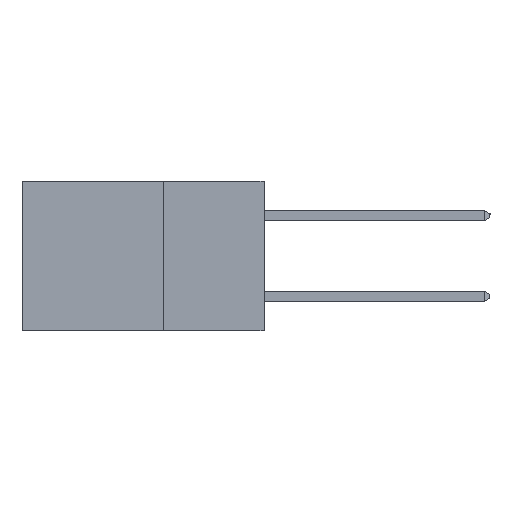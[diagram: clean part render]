
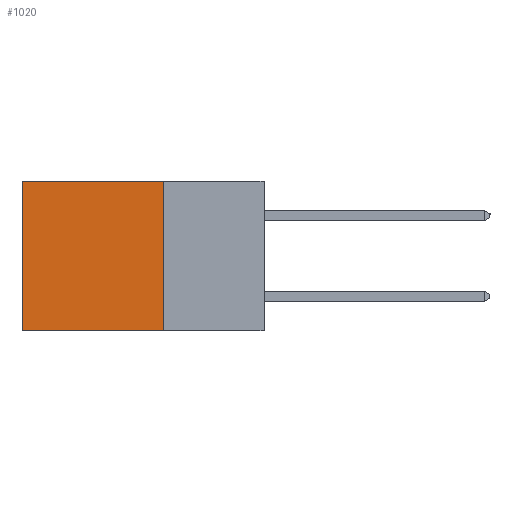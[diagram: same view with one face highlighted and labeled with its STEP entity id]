
A CAD part, left-side view. The second image highlights one B-rep face of the part: STEP entity #1020.
In plain terms, the highlighted planar face has unit normal (-1, 0, 0).
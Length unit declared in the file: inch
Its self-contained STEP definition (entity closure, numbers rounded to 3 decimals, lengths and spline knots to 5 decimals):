
#186 = VERTEX_POINT ( 'NONE', #15133 ) ;
#246 = VERTEX_POINT ( 'NONE', #11423 ) ;
#358 = AXIS2_PLACEMENT_3D ( 'NONE', #12783, #1730, #6645 ) ;
#474 = VECTOR ( 'NONE', #1845, 39.37008 ) ;
#616 = VECTOR ( 'NONE', #12439, 39.37008 ) ;
#1020 = ADVANCED_FACE ( 'NONE', ( #1878 ), #7836, .F. ) ;
#1242 = VECTOR ( 'NONE', #9492, 39.37008 ) ;
#1294 = EDGE_CURVE ( 'NONE', #246, #11935, #6142, .T. ) ;
#1351 = VERTEX_POINT ( 'NONE', #8967 ) ;
#1730 = DIRECTION ( 'NONE',  ( 1., 0., 0. ) ) ;
#1845 = DIRECTION ( 'NONE',  ( 0., 1., 0. ) ) ;
#1878 = FACE_OUTER_BOUND ( 'NONE', #4104, .T. ) ;
#2169 = CARTESIAN_POINT ( 'NONE',  ( 0.2615, 0.25, 0. ) ) ;
#2902 = EDGE_CURVE ( 'NONE', #186, #11935, #14388, .T. ) ;
#3236 = CARTESIAN_POINT ( 'NONE',  ( 0.2615, 0.6, -0.37 ) ) ;
#4104 = EDGE_LOOP ( 'NONE', ( #14423, #11786, #11296, #11541 ) ) ;
#4579 = CARTESIAN_POINT ( 'NONE',  ( 0.2615, 0.25, -0.37 ) ) ;
#6142 = LINE ( 'NONE', #7496, #616 ) ;
#6315 = EDGE_CURVE ( 'NONE', #1351, #186, #14202, .T. ) ;
#6562 = CARTESIAN_POINT ( 'NONE',  ( 0.2615, 0.6, -0.37 ) ) ;
#6645 = DIRECTION ( 'NONE',  ( 0., 0., -1. ) ) ;
#7496 = CARTESIAN_POINT ( 'NONE',  ( 0.2615, 0.25, -0.37 ) ) ;
#7836 = PLANE ( 'NONE',  #358 ) ;
#8222 = EDGE_CURVE ( 'NONE', #1351, #246, #15623, .T. ) ;
#8967 = CARTESIAN_POINT ( 'NONE',  ( 0.2615, 0.25, 0. ) ) ;
#9492 = DIRECTION ( 'NONE',  ( 0., 0., -1. ) ) ;
#11296 = ORIENTED_EDGE ( 'NONE', *, *, #8222, .F. ) ;
#11423 = CARTESIAN_POINT ( 'NONE',  ( 0.2615, 0.25, -0.37 ) ) ;
#11541 = ORIENTED_EDGE ( 'NONE', *, *, #6315, .T. ) ;
#11689 = VECTOR ( 'NONE', #11792, 39.37008 ) ;
#11786 = ORIENTED_EDGE ( 'NONE', *, *, #1294, .F. ) ;
#11792 = DIRECTION ( 'NONE',  ( 0., 0., -1. ) ) ;
#11935 = VERTEX_POINT ( 'NONE', #6562 ) ;
#12439 = DIRECTION ( 'NONE',  ( 0., 1., 0. ) ) ;
#12783 = CARTESIAN_POINT ( 'NONE',  ( 0.2615, 0.25, -0.37 ) ) ;
#14202 = LINE ( 'NONE', #2169, #474 ) ;
#14388 = LINE ( 'NONE', #3236, #11689 ) ;
#14423 = ORIENTED_EDGE ( 'NONE', *, *, #2902, .T. ) ;
#15133 = CARTESIAN_POINT ( 'NONE',  ( 0.2615, 0.6, 0. ) ) ;
#15623 = LINE ( 'NONE', #4579, #1242 ) ;
